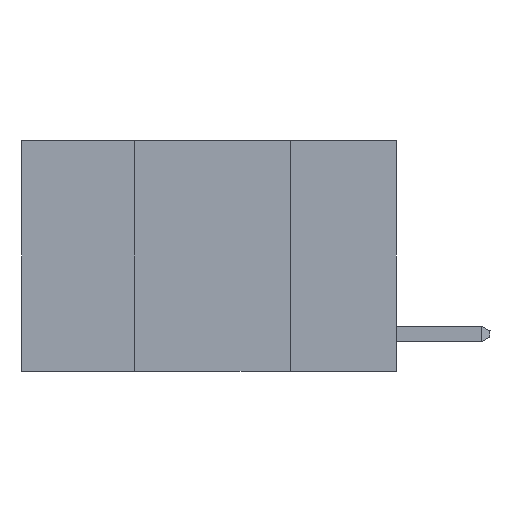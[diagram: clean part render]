
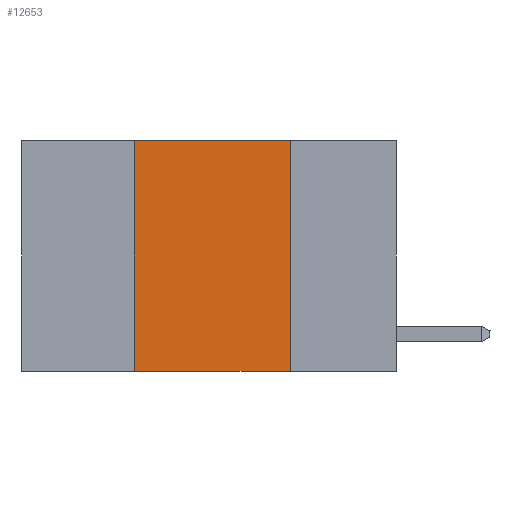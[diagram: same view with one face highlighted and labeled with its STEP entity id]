
A CAD part, left-side view. The second image highlights one B-rep face of the part: STEP entity #12653.
In plain terms, the highlighted planar face has unit normal (-1, 0, 0).
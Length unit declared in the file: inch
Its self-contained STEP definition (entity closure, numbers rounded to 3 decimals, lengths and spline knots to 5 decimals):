
#121 = VERTEX_POINT ( 'NONE', #10033 ) ;
#661 = CARTESIAN_POINT ( 'NONE',  ( 0., 0.6, -0.37 ) ) ;
#870 = ORIENTED_EDGE ( 'NONE', *, *, #7057, .F. ) ;
#1246 = LINE ( 'NONE', #661, #12143 ) ;
#1612 = LINE ( 'NONE', #17833, #8603 ) ;
#1617 = ORIENTED_EDGE ( 'NONE', *, *, #2172, .T. ) ;
#2172 = EDGE_CURVE ( 'NONE', #6064, #121, #1246, .T. ) ;
#2183 = AXIS2_PLACEMENT_3D ( 'NONE', #13891, #12452, #15678 ) ;
#2261 = CARTESIAN_POINT ( 'NONE',  ( 0., 0.17, 0. ) ) ;
#2476 = VECTOR ( 'NONE', #10897, 39.37008 ) ;
#3713 = ORIENTED_EDGE ( 'NONE', *, *, #12357, .F. ) ;
#3855 = CARTESIAN_POINT ( 'NONE',  ( 0., 0.17, 0. ) ) ;
#4676 = ORIENTED_EDGE ( 'NONE', *, *, #11106, .F. ) ;
#5255 = CARTESIAN_POINT ( 'NONE',  ( 0., 0.42, 0. ) ) ;
#5296 = FACE_OUTER_BOUND ( 'NONE', #16192, .T. ) ;
#5957 = VERTEX_POINT ( 'NONE', #5255 ) ;
#6064 = VERTEX_POINT ( 'NONE', #10943 ) ;
#6411 = DIRECTION ( 'NONE',  ( 0., -1., 0. ) ) ;
#6935 = VECTOR ( 'NONE', #7098, 39.37008 ) ;
#7057 = EDGE_CURVE ( 'NONE', #6064, #5957, #1612, .T. ) ;
#7098 = DIRECTION ( 'NONE',  ( 0., 0., -1. ) ) ;
#7472 = LINE ( 'NONE', #14862, #2476 ) ;
#8603 = VECTOR ( 'NONE', #12548, 39.37008 ) ;
#10033 = CARTESIAN_POINT ( 'NONE',  ( 0., 0.17, -0.37 ) ) ;
#10897 = DIRECTION ( 'NONE',  ( 0., -1., 0. ) ) ;
#10943 = CARTESIAN_POINT ( 'NONE',  ( 0., 0.42, -0.37 ) ) ;
#11106 = EDGE_CURVE ( 'NONE', #15118, #121, #15200, .T. ) ;
#12143 = VECTOR ( 'NONE', #6411, 39.37008 ) ;
#12357 = EDGE_CURVE ( 'NONE', #5957, #15118, #7472, .T. ) ;
#12452 = DIRECTION ( 'NONE',  ( 1., 0., 0. ) ) ;
#12548 = DIRECTION ( 'NONE',  ( 0., 0., 1. ) ) ;
#12653 = ADVANCED_FACE ( 'NONE', ( #5296 ), #14013, .F. ) ;
#13891 = CARTESIAN_POINT ( 'NONE',  ( 0., 0.6, 0. ) ) ;
#14013 = PLANE ( 'NONE',  #2183 ) ;
#14862 = CARTESIAN_POINT ( 'NONE',  ( 0., 0.6, 0. ) ) ;
#15118 = VERTEX_POINT ( 'NONE', #2261 ) ;
#15200 = LINE ( 'NONE', #3855, #6935 ) ;
#15678 = DIRECTION ( 'NONE',  ( 0., 0., -1. ) ) ;
#16192 = EDGE_LOOP ( 'NONE', ( #4676, #3713, #870, #1617 ) ) ;
#17833 = CARTESIAN_POINT ( 'NONE',  ( 0., 0.42, 0. ) ) ;
